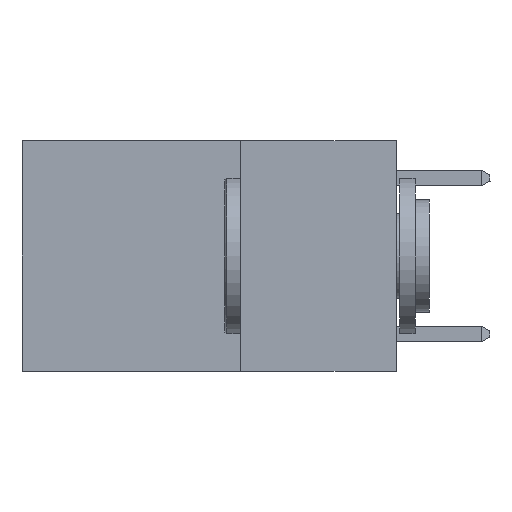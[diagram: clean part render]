
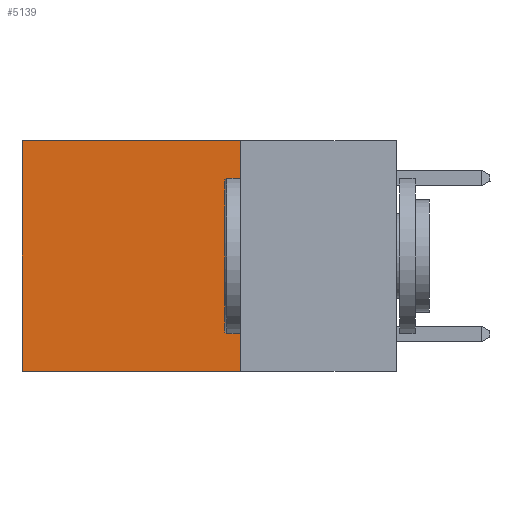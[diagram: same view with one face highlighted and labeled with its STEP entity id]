
A CAD part, left-side view. The second image highlights one B-rep face of the part: STEP entity #5139.
In plain terms, the highlighted planar face has unit normal (-1, 0, 0).
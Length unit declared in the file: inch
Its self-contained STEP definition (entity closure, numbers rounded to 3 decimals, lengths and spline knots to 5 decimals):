
#58 = EDGE_CURVE ( 'NONE', #2143, #5654, #6560, .T. ) ;
#754 = LINE ( 'NONE', #19195, #6773 ) ;
#899 = ORIENTED_EDGE ( 'NONE', *, *, #58, .F. ) ;
#2143 = VERTEX_POINT ( 'NONE', #5869 ) ;
#2427 = EDGE_LOOP ( 'NONE', ( #19752, #899, #18537, #20953 ) ) ;
#2852 = EDGE_CURVE ( 'NONE', #11652, #5654, #16007, .T. ) ;
#3685 = DIRECTION ( 'NONE',  ( 0., 1., 0. ) ) ;
#5139 = ADVANCED_FACE ( 'NONE', ( #7338 ), #19115, .F. ) ;
#5169 = EDGE_CURVE ( 'NONE', #9438, #11652, #754, .T. ) ;
#5564 = EDGE_CURVE ( 'NONE', #9438, #2143, #10447, .T. ) ;
#5654 = VERTEX_POINT ( 'NONE', #16677 ) ;
#5869 = CARTESIAN_POINT ( 'NONE',  ( 0.2625, 0.25, -0.37 ) ) ;
#6000 = AXIS2_PLACEMENT_3D ( 'NONE', #11536, #6272, #20689 ) ;
#6272 = DIRECTION ( 'NONE',  ( 1., 0., 0. ) ) ;
#6560 = LINE ( 'NONE', #12644, #20367 ) ;
#6773 = VECTOR ( 'NONE', #20990, 39.37008 ) ;
#7338 = FACE_OUTER_BOUND ( 'NONE', #2427, .T. ) ;
#7861 = CARTESIAN_POINT ( 'NONE',  ( 0.2625, 0.25, 0. ) ) ;
#8335 = CARTESIAN_POINT ( 'NONE',  ( 0.2625, 0.6, 0. ) ) ;
#9438 = VERTEX_POINT ( 'NONE', #7861 ) ;
#10447 = LINE ( 'NONE', #16107, #12161 ) ;
#11536 = CARTESIAN_POINT ( 'NONE',  ( 0.2625, 0.25, 0. ) ) ;
#11652 = VERTEX_POINT ( 'NONE', #17053 ) ;
#12161 = VECTOR ( 'NONE', #12494, 39.37008 ) ;
#12494 = DIRECTION ( 'NONE',  ( 0., 0., -1. ) ) ;
#12621 = DIRECTION ( 'NONE',  ( 0., 0., -1. ) ) ;
#12644 = CARTESIAN_POINT ( 'NONE',  ( 0.2625, 0.25, -0.37 ) ) ;
#16007 = LINE ( 'NONE', #8335, #16274 ) ;
#16107 = CARTESIAN_POINT ( 'NONE',  ( 0.2625, 0.25, 0. ) ) ;
#16274 = VECTOR ( 'NONE', #12621, 39.37008 ) ;
#16677 = CARTESIAN_POINT ( 'NONE',  ( 0.2625, 0.6, -0.37 ) ) ;
#17053 = CARTESIAN_POINT ( 'NONE',  ( 0.2625, 0.6, 0. ) ) ;
#18537 = ORIENTED_EDGE ( 'NONE', *, *, #5564, .F. ) ;
#19115 = PLANE ( 'NONE',  #6000 ) ;
#19195 = CARTESIAN_POINT ( 'NONE',  ( 0.2625, 0.25, 0. ) ) ;
#19752 = ORIENTED_EDGE ( 'NONE', *, *, #2852, .T. ) ;
#20367 = VECTOR ( 'NONE', #3685, 39.37008 ) ;
#20689 = DIRECTION ( 'NONE',  ( 0., 0., -1. ) ) ;
#20953 = ORIENTED_EDGE ( 'NONE', *, *, #5169, .T. ) ;
#20990 = DIRECTION ( 'NONE',  ( 0., 1., 0. ) ) ;
